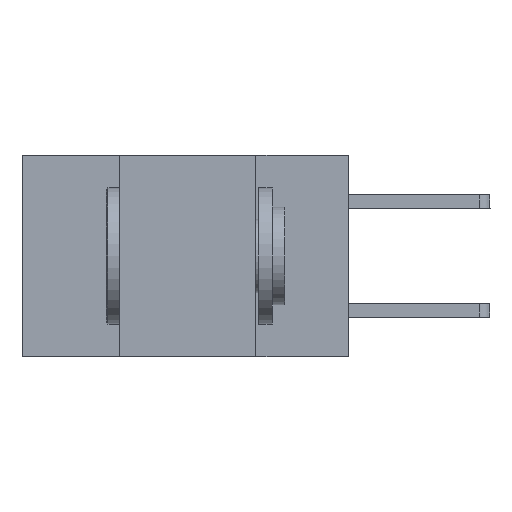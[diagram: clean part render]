
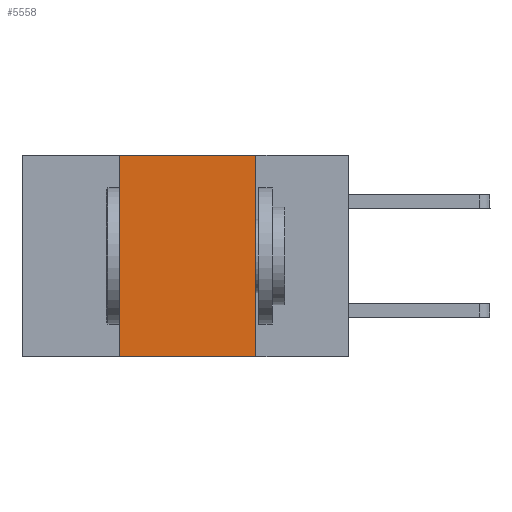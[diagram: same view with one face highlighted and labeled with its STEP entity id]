
A CAD part, left-side view. The second image highlights one B-rep face of the part: STEP entity #5558.
In plain terms, the highlighted planar face has unit normal (-1, 0, 0).
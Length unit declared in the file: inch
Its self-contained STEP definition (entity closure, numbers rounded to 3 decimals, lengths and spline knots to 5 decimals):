
#52 = LINE ( 'NONE', #7069, #6872 ) ;
#187 = EDGE_CURVE ( 'NONE', #7834, #6352, #5443, .T. ) ;
#219 = VERTEX_POINT ( 'NONE', #5336 ) ;
#789 = DIRECTION ( 'NONE',  ( 0., -1., 0. ) ) ;
#1221 = ORIENTED_EDGE ( 'NONE', *, *, #187, .T. ) ;
#1235 = ORIENTED_EDGE ( 'NONE', *, *, #4532, .F. ) ;
#1276 = PLANE ( 'NONE',  #9720 ) ;
#1718 = EDGE_CURVE ( 'NONE', #219, #7664, #2625, .T. ) ;
#2277 = DIRECTION ( 'NONE',  ( 1., 0., 0. ) ) ;
#2625 = LINE ( 'NONE', #5786, #3504 ) ;
#2639 = DIRECTION ( 'NONE',  ( 0., 0., -1. ) ) ;
#3504 = VECTOR ( 'NONE', #789, 39.37008 ) ;
#4249 = LINE ( 'NONE', #4353, #9538 ) ;
#4353 = CARTESIAN_POINT ( 'NONE',  ( 0., 0.17, -0.37 ) ) ;
#4405 = CARTESIAN_POINT ( 'NONE',  ( 0., 0.6, -0.37 ) ) ;
#4532 = EDGE_CURVE ( 'NONE', #7664, #6352, #4249, .T. ) ;
#4926 = EDGE_CURVE ( 'NONE', #7834, #219, #52, .T. ) ;
#5336 = CARTESIAN_POINT ( 'NONE',  ( 0., 0.42, 0. ) ) ;
#5416 = EDGE_LOOP ( 'NONE', ( #1235, #6798, #9339, #1221 ) ) ;
#5443 = LINE ( 'NONE', #4405, #7280 ) ;
#5558 = ADVANCED_FACE ( 'NONE', ( #9398 ), #1276, .F. ) ;
#5786 = CARTESIAN_POINT ( 'NONE',  ( 0., 0.6, 0. ) ) ;
#5792 = CARTESIAN_POINT ( 'NONE',  ( 0., 0.17, 0. ) ) ;
#6352 = VERTEX_POINT ( 'NONE', #9094 ) ;
#6470 = DIRECTION ( 'NONE',  ( 0., 0., 1. ) ) ;
#6798 = ORIENTED_EDGE ( 'NONE', *, *, #1718, .F. ) ;
#6872 = VECTOR ( 'NONE', #6470, 39.37008 ) ;
#7069 = CARTESIAN_POINT ( 'NONE',  ( 0., 0.42, -0.37 ) ) ;
#7280 = VECTOR ( 'NONE', #7547, 39.37008 ) ;
#7547 = DIRECTION ( 'NONE',  ( 0., -1., 0. ) ) ;
#7664 = VERTEX_POINT ( 'NONE', #5792 ) ;
#7834 = VERTEX_POINT ( 'NONE', #8887 ) ;
#8399 = DIRECTION ( 'NONE',  ( 0., 0., -1. ) ) ;
#8887 = CARTESIAN_POINT ( 'NONE',  ( 0., 0.42, -0.37 ) ) ;
#9094 = CARTESIAN_POINT ( 'NONE',  ( 0., 0.17, -0.37 ) ) ;
#9339 = ORIENTED_EDGE ( 'NONE', *, *, #4926, .F. ) ;
#9398 = FACE_OUTER_BOUND ( 'NONE', #5416, .T. ) ;
#9538 = VECTOR ( 'NONE', #2639, 39.37008 ) ;
#9720 = AXIS2_PLACEMENT_3D ( 'NONE', #10219, #2277, #8399 ) ;
#10219 = CARTESIAN_POINT ( 'NONE',  ( 0., 0.6, 0. ) ) ;
